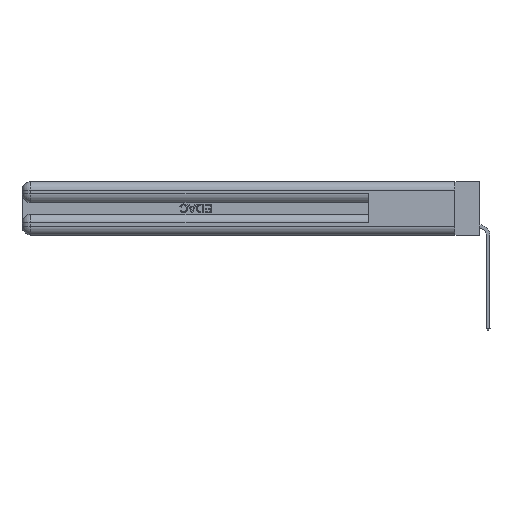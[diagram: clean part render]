
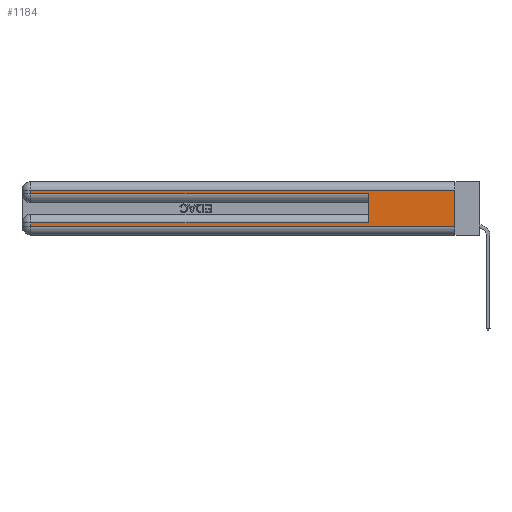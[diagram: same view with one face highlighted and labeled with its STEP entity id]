
A CAD part, left-side view. The second image highlights one B-rep face of the part: STEP entity #1184.
In plain terms, the highlighted planar face has unit normal (-1, 0, 0).
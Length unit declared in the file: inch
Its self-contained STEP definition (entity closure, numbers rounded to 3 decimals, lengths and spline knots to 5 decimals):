
#431 = DIRECTION ( 'NONE',  ( 0., 1., 0. ) ) ;
#500 = CARTESIAN_POINT ( 'NONE',  ( 0., 0.6, 0.285 ) ) ;
#569 = DIRECTION ( 'NONE',  ( 0., 0., -1. ) ) ;
#1114 = VECTOR ( 'NONE', #8355, 39.37008 ) ;
#1184 = ADVANCED_FACE ( 'NONE', ( #24184 ), #23492, .F. ) ;
#2120 = LINE ( 'NONE', #5164, #27946 ) ;
#2176 = EDGE_LOOP ( 'NONE', ( #15662, #14958, #29626, #26473, #29729, #11555, #20613, #28779 ) ) ;
#2212 = CARTESIAN_POINT ( 'NONE',  ( 0., 0., 0.06 ) ) ;
#2471 = EDGE_CURVE ( 'NONE', #26226, #6285, #31368, .T. ) ;
#2627 = CARTESIAN_POINT ( 'NONE',  ( 0., 0., 0.285 ) ) ;
#2688 = VERTEX_POINT ( 'NONE', #15927 ) ;
#2740 = CARTESIAN_POINT ( 'NONE',  ( 0., 0., 0.06 ) ) ;
#4056 = DIRECTION ( 'NONE',  ( 0., 0., -1. ) ) ;
#4628 = DIRECTION ( 'NONE',  ( 0., -1., 0. ) ) ;
#4670 = VECTOR ( 'NONE', #14703, 39.37008 ) ;
#5164 = CARTESIAN_POINT ( 'NONE',  ( 0., 0., 0.085 ) ) ;
#6285 = VERTEX_POINT ( 'NONE', #28136 ) ;
#7528 = LINE ( 'NONE', #30143, #1114 ) ;
#7880 = DIRECTION ( 'NONE',  ( 0., 1., 0. ) ) ;
#7906 = EDGE_CURVE ( 'NONE', #2688, #14676, #9620, .T. ) ;
#8285 = EDGE_CURVE ( 'NONE', #11656, #14676, #30558, .T. ) ;
#8355 = DIRECTION ( 'NONE',  ( 0., 0., -1. ) ) ;
#9022 = VECTOR ( 'NONE', #4628, 39.37008 ) ;
#9347 = VECTOR ( 'NONE', #569, 39.37008 ) ;
#9620 = LINE ( 'NONE', #28056, #21036 ) ;
#10613 = EDGE_CURVE ( 'NONE', #2688, #17928, #2120, .T. ) ;
#11555 = ORIENTED_EDGE ( 'NONE', *, *, #10613, .T. ) ;
#11656 = VERTEX_POINT ( 'NONE', #30553 ) ;
#13469 = DIRECTION ( 'NONE',  ( 0., 0., 1. ) ) ;
#14676 = VERTEX_POINT ( 'NONE', #500 ) ;
#14703 = DIRECTION ( 'NONE',  ( 0., -1., 0. ) ) ;
#14958 = ORIENTED_EDGE ( 'NONE', *, *, #2471, .T. ) ;
#15067 = CARTESIAN_POINT ( 'NONE',  ( 0., 0., 0.31 ) ) ;
#15268 = DIRECTION ( 'NONE',  ( 0., 0., -1. ) ) ;
#15465 = AXIS2_PLACEMENT_3D ( 'NONE', #30863, #30083, #4056 ) ;
#15662 = ORIENTED_EDGE ( 'NONE', *, *, #18693, .F. ) ;
#15892 = EDGE_CURVE ( 'NONE', #25249, #18478, #21167, .T. ) ;
#15927 = CARTESIAN_POINT ( 'NONE',  ( 0., 0.6, 0.085 ) ) ;
#16761 = EDGE_CURVE ( 'NONE', #17928, #25249, #17918, .T. ) ;
#17602 = CARTESIAN_POINT ( 'NONE',  ( 0., 2.94, 0.37 ) ) ;
#17918 = LINE ( 'NONE', #17602, #30114 ) ;
#17928 = VERTEX_POINT ( 'NONE', #27337 ) ;
#18391 = VECTOR ( 'NONE', #7880, 39.37008 ) ;
#18478 = VERTEX_POINT ( 'NONE', #2740 ) ;
#18693 = EDGE_CURVE ( 'NONE', #26226, #18478, #7528, .T. ) ;
#20613 = ORIENTED_EDGE ( 'NONE', *, *, #16761, .T. ) ;
#20720 = CARTESIAN_POINT ( 'NONE',  ( 0., 0., 0.31 ) ) ;
#21036 = VECTOR ( 'NONE', #13469, 39.37008 ) ;
#21167 = LINE ( 'NONE', #2212, #9022 ) ;
#23492 = PLANE ( 'NONE',  #15465 ) ;
#24184 = FACE_OUTER_BOUND ( 'NONE', #2176, .T. ) ;
#25249 = VERTEX_POINT ( 'NONE', #28958 ) ;
#26226 = VERTEX_POINT ( 'NONE', #20720 ) ;
#26473 = ORIENTED_EDGE ( 'NONE', *, *, #8285, .T. ) ;
#27337 = CARTESIAN_POINT ( 'NONE',  ( 0., 2.94, 0.085 ) ) ;
#27526 = EDGE_CURVE ( 'NONE', #6285, #11656, #28758, .T. ) ;
#27946 = VECTOR ( 'NONE', #431, 39.37008 ) ;
#28056 = CARTESIAN_POINT ( 'NONE',  ( 0., 0.6, 0.145 ) ) ;
#28136 = CARTESIAN_POINT ( 'NONE',  ( 0., 2.94, 0.31 ) ) ;
#28758 = LINE ( 'NONE', #29634, #9347 ) ;
#28779 = ORIENTED_EDGE ( 'NONE', *, *, #15892, .T. ) ;
#28958 = CARTESIAN_POINT ( 'NONE',  ( 0., 2.94, 0.06 ) ) ;
#29626 = ORIENTED_EDGE ( 'NONE', *, *, #27526, .T. ) ;
#29634 = CARTESIAN_POINT ( 'NONE',  ( 0., 2.94, 0.37 ) ) ;
#29729 = ORIENTED_EDGE ( 'NONE', *, *, #7906, .F. ) ;
#30083 = DIRECTION ( 'NONE',  ( 1., 0., 0. ) ) ;
#30114 = VECTOR ( 'NONE', #15268, 39.37008 ) ;
#30143 = CARTESIAN_POINT ( 'NONE',  ( 0., 0., 0.37 ) ) ;
#30553 = CARTESIAN_POINT ( 'NONE',  ( 0., 2.94, 0.285 ) ) ;
#30558 = LINE ( 'NONE', #2627, #4670 ) ;
#30863 = CARTESIAN_POINT ( 'NONE',  ( 0., 0., 0.37 ) ) ;
#31368 = LINE ( 'NONE', #15067, #18391 ) ;
